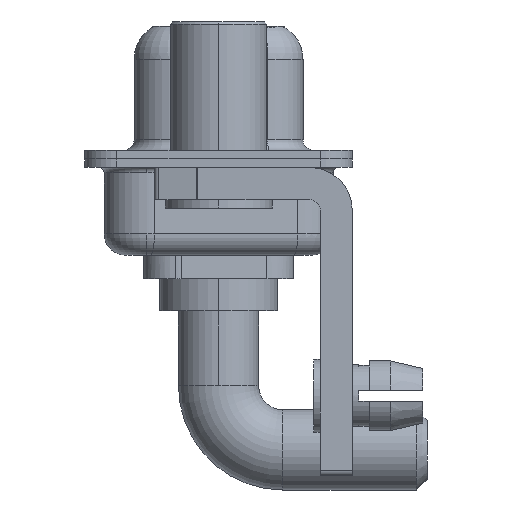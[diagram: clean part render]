
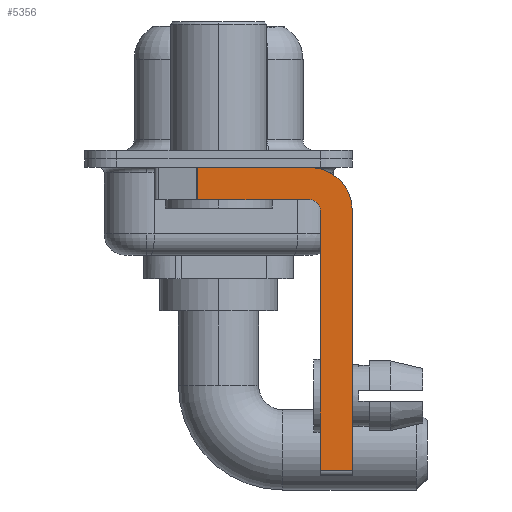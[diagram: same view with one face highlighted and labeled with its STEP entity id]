
A CAD part, left-side view. The second image highlights one B-rep face of the part: STEP entity #5356.
In plain terms, the highlighted planar face has unit normal (-1, 0, 0).
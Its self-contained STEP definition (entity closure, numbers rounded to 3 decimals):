
#64 = EDGE_CURVE ( 'NONE', #1626, #789, #16760, .T. ) ;
#416 = PLANE ( 'NONE',  #5028 ) ;
#789 = VERTEX_POINT ( 'NONE', #10716 ) ;
#814 = CARTESIAN_POINT ( 'NONE',  ( -2.9, 3., -0.4 ) ) ;
#1105 = CARTESIAN_POINT ( 'NONE',  ( -2.9, -4.25, -1.9 ) ) ;
#1142 = VERTEX_POINT ( 'NONE', #7823 ) ;
#1626 = VERTEX_POINT ( 'NONE', #15625 ) ;
#1893 = EDGE_CURVE ( 'NONE', #5274, #5436, #10611, .T. ) ;
#2735 = CARTESIAN_POINT ( 'NONE',  ( -2.9, -6.25, -2.4 ) ) ;
#3191 = LINE ( 'NONE', #9653, #5285 ) ;
#3673 = DIRECTION ( 'NONE',  ( 0., 0., -1. ) ) ;
#4444 = EDGE_LOOP ( 'NONE', ( #15137, #15270, #11416, #7801, #7043, #7986, #5173, #14354 ) ) ;
#4512 = DIRECTION ( 'NONE',  ( 0., 1., 0. ) ) ;
#4570 = EDGE_CURVE ( 'NONE', #1626, #16838, #16233, .T. ) ;
#4597 = LINE ( 'NONE', #8661, #5021 ) ;
#4757 = DIRECTION ( 'NONE',  ( 0., -1., 0. ) ) ;
#4784 = EDGE_CURVE ( 'NONE', #7214, #1142, #3191, .T. ) ;
#4818 = CARTESIAN_POINT ( 'NONE',  ( -2.9, -4.75, -14.8 ) ) ;
#4952 = CARTESIAN_POINT ( 'NONE',  ( -2.9, -4.25, -0.4 ) ) ;
#5021 = VECTOR ( 'NONE', #4512, 1000. ) ;
#5028 = AXIS2_PLACEMENT_3D ( 'NONE', #13969, #9863, #8844 ) ;
#5114 = EDGE_CURVE ( 'NONE', #6450, #1142, #9034, .T. ) ;
#5173 = ORIENTED_EDGE ( 'NONE', *, *, #5114, .F. ) ;
#5274 = VERTEX_POINT ( 'NONE', #9779 ) ;
#5285 = VECTOR ( 'NONE', #6792, 1000. ) ;
#5302 = DIRECTION ( 'NONE',  ( 1., 0., 0. ) ) ;
#5356 = ADVANCED_FACE ( 'NONE', ( #5875 ), #416, .F. ) ;
#5436 = VERTEX_POINT ( 'NONE', #1105 ) ;
#5875 = FACE_OUTER_BOUND ( 'NONE', #4444, .T. ) ;
#5949 = VECTOR ( 'NONE', #3673, 1000. ) ;
#6450 = VERTEX_POINT ( 'NONE', #10785 ) ;
#6669 = DIRECTION ( 'NONE',  ( 0., 0., -1. ) ) ;
#6792 = DIRECTION ( 'NONE',  ( 0., -1., 0. ) ) ;
#7043 = ORIENTED_EDGE ( 'NONE', *, *, #14676, .F. ) ;
#7214 = VERTEX_POINT ( 'NONE', #14952 ) ;
#7801 = ORIENTED_EDGE ( 'NONE', *, *, #1893, .F. ) ;
#7816 = VECTOR ( 'NONE', #15193, 1000. ) ;
#7823 = CARTESIAN_POINT ( 'NONE',  ( -2.9, -6.25, -14.55 ) ) ;
#7986 = ORIENTED_EDGE ( 'NONE', *, *, #4784, .T. ) ;
#8110 = DIRECTION ( 'NONE',  ( -1., 0., 0. ) ) ;
#8661 = CARTESIAN_POINT ( 'NONE',  ( -2.9, -4.25, -1.9 ) ) ;
#8764 = CARTESIAN_POINT ( 'NONE',  ( -2.9, 0.978, -1.9 ) ) ;
#8784 = AXIS2_PLACEMENT_3D ( 'NONE', #16684, #5302, #11754 ) ;
#8844 = DIRECTION ( 'NONE',  ( 0., 0., -1. ) ) ;
#9034 = LINE ( 'NONE', #2735, #9070 ) ;
#9070 = VECTOR ( 'NONE', #6669, 1000. ) ;
#9653 = CARTESIAN_POINT ( 'NONE',  ( -2.9, -4.25, -14.55 ) ) ;
#9779 = CARTESIAN_POINT ( 'NONE',  ( -2.9, -4.75, -2.4 ) ) ;
#9863 = DIRECTION ( 'NONE',  ( 1., 0., 0. ) ) ;
#10611 = CIRCLE ( 'NONE', #16315, 0.5 ) ;
#10716 = CARTESIAN_POINT ( 'NONE',  ( -2.9, 0.978, -1.9 ) ) ;
#10785 = CARTESIAN_POINT ( 'NONE',  ( -2.9, -6.25, -2.4 ) ) ;
#11416 = ORIENTED_EDGE ( 'NONE', *, *, #13351, .F. ) ;
#11754 = DIRECTION ( 'NONE',  ( 0., 0., -1. ) ) ;
#12060 = CIRCLE ( 'NONE', #8784, 2. ) ;
#13028 = EDGE_CURVE ( 'NONE', #16838, #6450, #12060, .T. ) ;
#13351 = EDGE_CURVE ( 'NONE', #5436, #789, #4597, .T. ) ;
#13472 = CARTESIAN_POINT ( 'NONE',  ( -2.9, -4.25, -2.4 ) ) ;
#13969 = CARTESIAN_POINT ( 'NONE',  ( -2.9, -4.25, -2.4 ) ) ;
#14004 = LINE ( 'NONE', #4818, #7816 ) ;
#14233 = VECTOR ( 'NONE', #4757, 1000. ) ;
#14354 = ORIENTED_EDGE ( 'NONE', *, *, #13028, .F. ) ;
#14676 = EDGE_CURVE ( 'NONE', #7214, #5274, #14004, .T. ) ;
#14952 = CARTESIAN_POINT ( 'NONE',  ( -2.9, -4.75, -14.55 ) ) ;
#15137 = ORIENTED_EDGE ( 'NONE', *, *, #4570, .F. ) ;
#15193 = DIRECTION ( 'NONE',  ( 0., 0., 1. ) ) ;
#15270 = ORIENTED_EDGE ( 'NONE', *, *, #64, .T. ) ;
#15625 = CARTESIAN_POINT ( 'NONE',  ( -2.9, 0.978, -0.4 ) ) ;
#16029 = DIRECTION ( 'NONE',  ( 0., 0., 1. ) ) ;
#16233 = LINE ( 'NONE', #814, #14233 ) ;
#16315 = AXIS2_PLACEMENT_3D ( 'NONE', #13472, #8110, #16029 ) ;
#16684 = CARTESIAN_POINT ( 'NONE',  ( -2.9, -4.25, -2.4 ) ) ;
#16760 = LINE ( 'NONE', #8764, #5949 ) ;
#16838 = VERTEX_POINT ( 'NONE', #4952 ) ;
